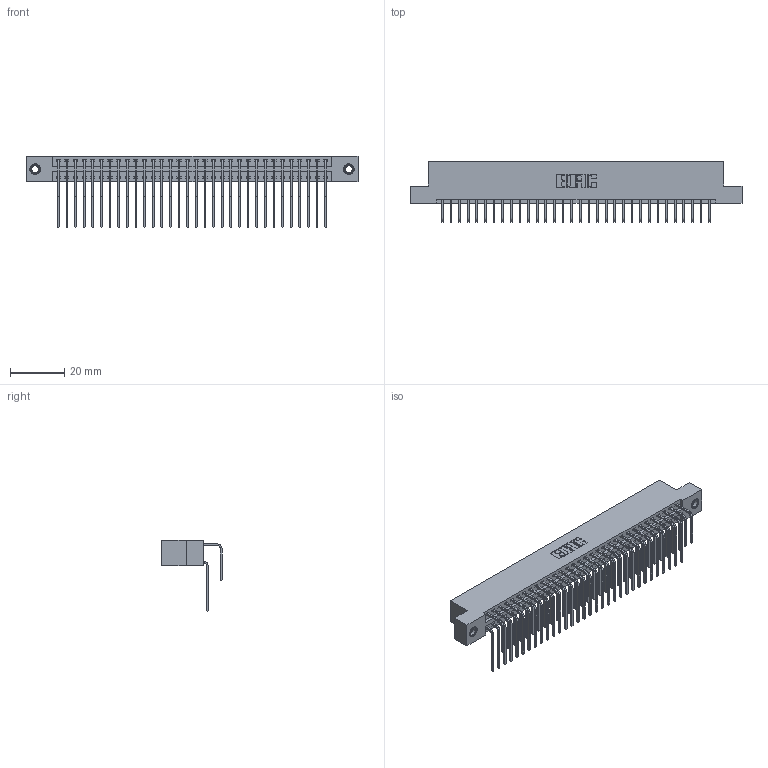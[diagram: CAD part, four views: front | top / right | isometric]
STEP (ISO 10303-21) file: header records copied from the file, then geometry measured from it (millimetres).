
FILE_DESCRIPTION (( 'STEP AP203' ), '1' );
FILE_NAME ('396-064-558-207.STEP', '2018-09-08T17:51:09', ( '' ), ( '' ), 'SwSTEP 2.0', 'SolidWorks 2016', '' );
FILE_SCHEMA (( 'CONFIG_CONTROL_DESIGN' ));
Length unit declared in the file: inch
Products named in the file (5): 396-064-558-207; 346 Part_Flush Mounting Lugs - 0.156 Dia-TI; 345-292-001_558 559 Tail - 1; 345-292-001_558 Tail - 2; 345-250-001_345-250-005-103
Assembly tree (67 placements, depth 2):
  396-064-558-207
    346 Part_Flush Mounting Lugs - 0.156 Dia-TI
    345-292-001_558 559 Tail - 1  x32
    345-292-001_558 Tail - 2  x32
    345-250-001_345-250-005-103  x2
Bounding box: 122.17 x 22.16 x 26.16 mm (x, y, z)
Volume: 12191.5 mm3; surface area: 18405.8 mm2
Topology: 67 solids, 67 shells, 3638 faces, 10769 edges, 7086 vertices
Faces by surface type: plane 2476, cylinder 1146, cone 12, torus 4
Entity records: 25200 total; most frequent: CARTESIAN_POINT 4202, ORIENTED_EDGE 4078, DIRECTION 3753, EDGE_CURVE 2039, LINE 1719, VECTOR 1719, VERTEX_POINT 1352, AXIS2_PLACEMENT_3D 1017
